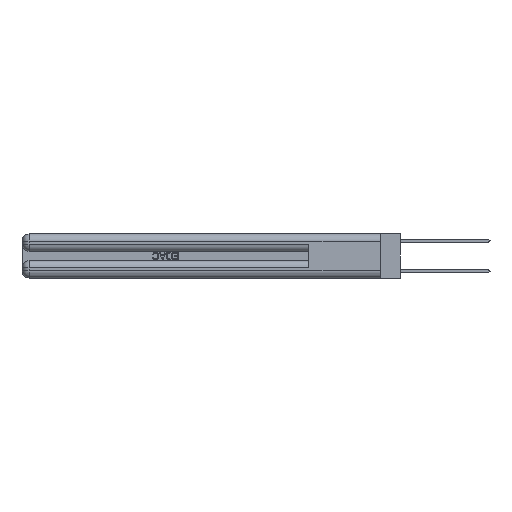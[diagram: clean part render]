
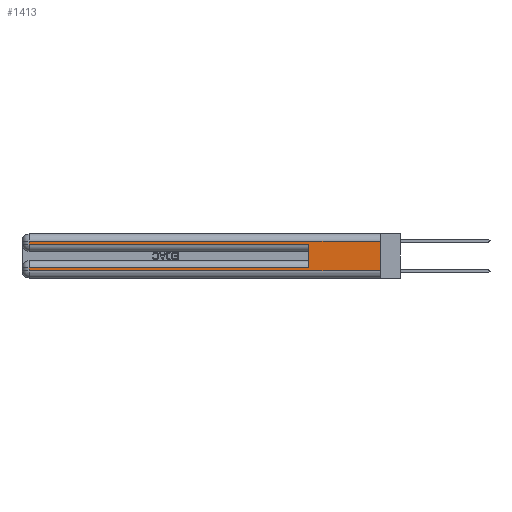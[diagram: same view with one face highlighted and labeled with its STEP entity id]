
A CAD part, left-side view. The second image highlights one B-rep face of the part: STEP entity #1413.
In plain terms, the highlighted planar face has unit normal (-1, 0, 0).
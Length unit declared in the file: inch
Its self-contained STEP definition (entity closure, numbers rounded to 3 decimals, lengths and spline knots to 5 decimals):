
#353 = ORIENTED_EDGE ( 'NONE', *, *, #21949, .F. ) ;
#426 = LINE ( 'NONE', #13413, #20155 ) ;
#1176 = DIRECTION ( 'NONE',  ( 0., 0., -1. ) ) ;
#1184 = EDGE_CURVE ( 'NONE', #19406, #18152, #23218, .T. ) ;
#1332 = ORIENTED_EDGE ( 'NONE', *, *, #10565, .F. ) ;
#1413 = ADVANCED_FACE ( 'NONE', ( #12759 ), #5117, .F. ) ;
#1889 = DIRECTION ( 'NONE',  ( 0., 0., -1. ) ) ;
#2243 = DIRECTION ( 'NONE',  ( 0., -1., 0. ) ) ;
#2327 = LINE ( 'NONE', #29598, #7010 ) ;
#2471 = DIRECTION ( 'NONE',  ( 0., 1., 0. ) ) ;
#2828 = VECTOR ( 'NONE', #1176, 39.37008 ) ;
#2972 = AXIS2_PLACEMENT_3D ( 'NONE', #16509, #9717, #25731 ) ;
#3244 = CARTESIAN_POINT ( 'NONE',  ( 0., 2.94, 0.285 ) ) ;
#3381 = ORIENTED_EDGE ( 'NONE', *, *, #1184, .T. ) ;
#4403 = ORIENTED_EDGE ( 'NONE', *, *, #11358, .T. ) ;
#5117 = PLANE ( 'NONE',  #2972 ) ;
#5134 = CARTESIAN_POINT ( 'NONE',  ( 0., 0.6, 0.085 ) ) ;
#6270 = VECTOR ( 'NONE', #2243, 39.37008 ) ;
#6276 = VERTEX_POINT ( 'NONE', #21808 ) ;
#6421 = VERTEX_POINT ( 'NONE', #21839 ) ;
#7010 = VECTOR ( 'NONE', #18180, 39.37008 ) ;
#7343 = CARTESIAN_POINT ( 'NONE',  ( 0., 0.6, 0.285 ) ) ;
#8160 = CARTESIAN_POINT ( 'NONE',  ( 0., 2.94, 0.06 ) ) ;
#8572 = VERTEX_POINT ( 'NONE', #13385 ) ;
#9590 = ORIENTED_EDGE ( 'NONE', *, *, #28175, .T. ) ;
#9717 = DIRECTION ( 'NONE',  ( 1., 0., 0. ) ) ;
#10365 = EDGE_CURVE ( 'NONE', #15604, #22745, #12263, .T. ) ;
#10565 = EDGE_CURVE ( 'NONE', #25624, #22745, #426, .T. ) ;
#10772 = VECTOR ( 'NONE', #2471, 39.37008 ) ;
#11358 = EDGE_CURVE ( 'NONE', #25624, #19406, #16142, .T. ) ;
#12263 = LINE ( 'NONE', #17328, #23752 ) ;
#12759 = FACE_OUTER_BOUND ( 'NONE', #16812, .T. ) ;
#13069 = LINE ( 'NONE', #22810, #6270 ) ;
#13385 = CARTESIAN_POINT ( 'NONE',  ( 0., 0., 0.31 ) ) ;
#13409 = ORIENTED_EDGE ( 'NONE', *, *, #10365, .T. ) ;
#13413 = CARTESIAN_POINT ( 'NONE',  ( 0., 0.6, 0.145 ) ) ;
#14067 = CARTESIAN_POINT ( 'NONE',  ( 0., 0., 0.31 ) ) ;
#15604 = VERTEX_POINT ( 'NONE', #3244 ) ;
#15718 = LINE ( 'NONE', #24050, #2828 ) ;
#15721 = DIRECTION ( 'NONE',  ( 0., 0., 1. ) ) ;
#16142 = LINE ( 'NONE', #23135, #10772 ) ;
#16370 = DIRECTION ( 'NONE',  ( 0., 1., 0. ) ) ;
#16509 = CARTESIAN_POINT ( 'NONE',  ( 0., 0., 0.37 ) ) ;
#16812 = EDGE_LOOP ( 'NONE', ( #353, #28769, #9590, #13409, #1332, #4403, #3381, #23473 ) ) ;
#17079 = VECTOR ( 'NONE', #1889, 39.37008 ) ;
#17328 = CARTESIAN_POINT ( 'NONE',  ( 0., 0., 0.285 ) ) ;
#18152 = VERTEX_POINT ( 'NONE', #8160 ) ;
#18180 = DIRECTION ( 'NONE',  ( 0., 0., -1. ) ) ;
#19406 = VERTEX_POINT ( 'NONE', #22825 ) ;
#19660 = DIRECTION ( 'NONE',  ( 0., -1., 0. ) ) ;
#20155 = VECTOR ( 'NONE', #15721, 39.37008 ) ;
#21808 = CARTESIAN_POINT ( 'NONE',  ( 0., 2.94, 0.31 ) ) ;
#21839 = CARTESIAN_POINT ( 'NONE',  ( 0., 0., 0.06 ) ) ;
#21949 = EDGE_CURVE ( 'NONE', #8572, #6421, #2327, .T. ) ;
#21975 = EDGE_CURVE ( 'NONE', #18152, #6421, #13069, .T. ) ;
#22745 = VERTEX_POINT ( 'NONE', #7343 ) ;
#22810 = CARTESIAN_POINT ( 'NONE',  ( 0., 0., 0.06 ) ) ;
#22825 = CARTESIAN_POINT ( 'NONE',  ( 0., 2.94, 0.085 ) ) ;
#23135 = CARTESIAN_POINT ( 'NONE',  ( 0., 0., 0.085 ) ) ;
#23218 = LINE ( 'NONE', #27036, #17079 ) ;
#23473 = ORIENTED_EDGE ( 'NONE', *, *, #21975, .T. ) ;
#23752 = VECTOR ( 'NONE', #19660, 39.37008 ) ;
#24050 = CARTESIAN_POINT ( 'NONE',  ( 0., 2.94, 0.37 ) ) ;
#25624 = VERTEX_POINT ( 'NONE', #5134 ) ;
#25731 = DIRECTION ( 'NONE',  ( 0., 0., -1. ) ) ;
#26945 = LINE ( 'NONE', #14067, #27677 ) ;
#27036 = CARTESIAN_POINT ( 'NONE',  ( 0., 2.94, 0.37 ) ) ;
#27677 = VECTOR ( 'NONE', #16370, 39.37008 ) ;
#28175 = EDGE_CURVE ( 'NONE', #6276, #15604, #15718, .T. ) ;
#28769 = ORIENTED_EDGE ( 'NONE', *, *, #29099, .T. ) ;
#29099 = EDGE_CURVE ( 'NONE', #8572, #6276, #26945, .T. ) ;
#29598 = CARTESIAN_POINT ( 'NONE',  ( 0., 0., 0.37 ) ) ;
